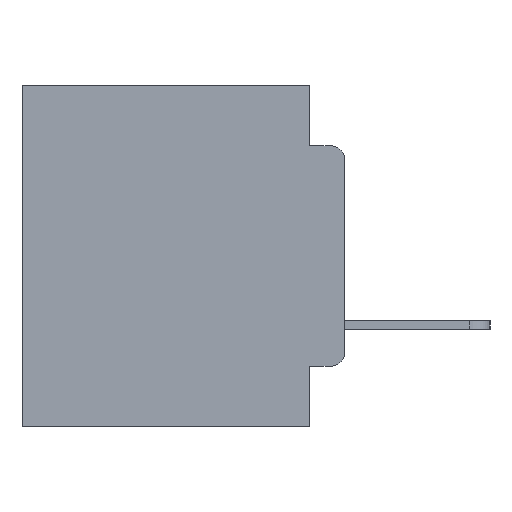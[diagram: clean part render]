
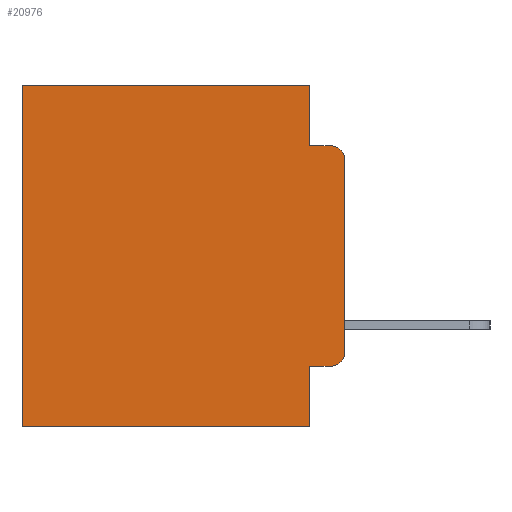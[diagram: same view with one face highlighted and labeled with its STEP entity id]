
A CAD part, left-side view. The second image highlights one B-rep face of the part: STEP entity #20976.
In plain terms, the highlighted planar face has unit normal (-1, 0, 0).
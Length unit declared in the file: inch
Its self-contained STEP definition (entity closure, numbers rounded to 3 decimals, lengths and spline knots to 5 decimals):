
#806 = CARTESIAN_POINT ( 'NONE',  ( 0.298, 0.051, -0.4115 ) ) ;
#814 = EDGE_LOOP ( 'NONE', ( #24958, #14508, #8921, #24069, #3174, #27564, #15172, #28397, #24677, #23780 ) ) ;
#1086 = VERTEX_POINT ( 'NONE', #5333 ) ;
#1125 = LINE ( 'NONE', #21818, #23109 ) ;
#1185 = DIRECTION ( 'NONE',  ( 0., 0., -1. ) ) ;
#1727 = DIRECTION ( 'NONE',  ( 1., 0., 0. ) ) ;
#2518 = CARTESIAN_POINT ( 'NONE',  ( 0.298, 0.051, -0.0885 ) ) ;
#2690 = VECTOR ( 'NONE', #19543, 39.37008 ) ;
#2940 = CARTESIAN_POINT ( 'NONE',  ( 0.298, 0., -0.1085 ) ) ;
#3174 = ORIENTED_EDGE ( 'NONE', *, *, #16804, .T. ) ;
#3252 = CARTESIAN_POINT ( 'NONE',  ( 0.298, 0.051, -0.0885 ) ) ;
#3328 = DIRECTION ( 'NONE',  ( 0., 0., -1. ) ) ;
#3521 = CARTESIAN_POINT ( 'NONE',  ( 0.298, 0., 0. ) ) ;
#3951 = CARTESIAN_POINT ( 'NONE',  ( 0.298, 0., 0. ) ) ;
#4166 = DIRECTION ( 'NONE',  ( 0., 0., -1. ) ) ;
#4371 = DIRECTION ( 'NONE',  ( 0., 1., 0. ) ) ;
#4729 = DIRECTION ( 'NONE',  ( 0., -1., 0. ) ) ;
#4752 = LINE ( 'NONE', #21910, #2690 ) ;
#4951 = EDGE_CURVE ( 'NONE', #8878, #1086, #20096, .T. ) ;
#5032 = DIRECTION ( 'NONE',  ( 0., -1., 0. ) ) ;
#5333 = CARTESIAN_POINT ( 'NONE',  ( 0.298, 0.02, -0.0885 ) ) ;
#6198 = LINE ( 'NONE', #19622, #10331 ) ;
#6362 = EDGE_CURVE ( 'NONE', #19296, #1086, #15864, .T. ) ;
#6628 = VECTOR ( 'NONE', #4371, 39.37008 ) ;
#6692 = EDGE_CURVE ( 'NONE', #16845, #23964, #1125, .T. ) ;
#7140 = AXIS2_PLACEMENT_3D ( 'NONE', #14344, #10156, #1185 ) ;
#7438 = AXIS2_PLACEMENT_3D ( 'NONE', #3951, #1727, #10714 ) ;
#7787 = CARTESIAN_POINT ( 'NONE',  ( 0.298, 0.051, -0.4115 ) ) ;
#7881 = EDGE_CURVE ( 'NONE', #19242, #22658, #18175, .T. ) ;
#8309 = VERTEX_POINT ( 'NONE', #23051 ) ;
#8380 = LINE ( 'NONE', #27489, #21716 ) ;
#8697 = AXIS2_PLACEMENT_3D ( 'NONE', #27974, #12816, #14950 ) ;
#8708 = DIRECTION ( 'NONE',  ( 0., 0., -1. ) ) ;
#8878 = VERTEX_POINT ( 'NONE', #2940 ) ;
#8921 = ORIENTED_EDGE ( 'NONE', *, *, #6362, .F. ) ;
#9061 = VECTOR ( 'NONE', #5032, 39.37008 ) ;
#9118 = FACE_OUTER_BOUND ( 'NONE', #814, .T. ) ;
#9378 = VECTOR ( 'NONE', #4729, 39.37008 ) ;
#10156 = DIRECTION ( 'NONE',  ( -1., 0., 0. ) ) ;
#10197 = EDGE_CURVE ( 'NONE', #8878, #22658, #28335, .T. ) ;
#10331 = VECTOR ( 'NONE', #8708, 39.37008 ) ;
#10714 = DIRECTION ( 'NONE',  ( 0., 0., -1. ) ) ;
#11926 = EDGE_CURVE ( 'NONE', #16845, #19242, #14888, .T. ) ;
#12172 = EDGE_CURVE ( 'NONE', #23964, #8309, #8380, .T. ) ;
#12650 = DIRECTION ( 'NONE',  ( 0., 1., 0. ) ) ;
#12816 = DIRECTION ( 'NONE',  ( -1., 0., 0. ) ) ;
#14344 = CARTESIAN_POINT ( 'NONE',  ( 0.298, 0.02, -0.1085 ) ) ;
#14508 = ORIENTED_EDGE ( 'NONE', *, *, #4951, .T. ) ;
#14625 = VECTOR ( 'NONE', #3328, 39.37008 ) ;
#14888 = LINE ( 'NONE', #806, #9061 ) ;
#14950 = DIRECTION ( 'NONE',  ( 0., 0., -1. ) ) ;
#15172 = ORIENTED_EDGE ( 'NONE', *, *, #12172, .F. ) ;
#15430 = CARTESIAN_POINT ( 'NONE',  ( 0.298, 0., -0.3915 ) ) ;
#15864 = LINE ( 'NONE', #2518, #9378 ) ;
#16404 = VERTEX_POINT ( 'NONE', #23049 ) ;
#16804 = EDGE_CURVE ( 'NONE', #16404, #25342, #20676, .T. ) ;
#16845 = VERTEX_POINT ( 'NONE', #7787 ) ;
#18175 = CIRCLE ( 'NONE', #8697, 0.02 ) ;
#19242 = VERTEX_POINT ( 'NONE', #20844 ) ;
#19296 = VERTEX_POINT ( 'NONE', #3252 ) ;
#19543 = DIRECTION ( 'NONE',  ( 0., 0., -1. ) ) ;
#19622 = CARTESIAN_POINT ( 'NONE',  ( 0.298, 0.473, 0. ) ) ;
#19835 = CARTESIAN_POINT ( 'NONE',  ( 0.298, 0., 0. ) ) ;
#20096 = CIRCLE ( 'NONE', #7140, 0.02 ) ;
#20669 = CARTESIAN_POINT ( 'NONE',  ( 0.298, 0.473, 0. ) ) ;
#20676 = LINE ( 'NONE', #19835, #6628 ) ;
#20844 = CARTESIAN_POINT ( 'NONE',  ( 0.298, 0.02, -0.4115 ) ) ;
#20976 = ADVANCED_FACE ( 'NONE', ( #9118 ), #26073, .F. ) ;
#21716 = VECTOR ( 'NONE', #12650, 39.37008 ) ;
#21818 = CARTESIAN_POINT ( 'NONE',  ( 0.298, 0.051, 0. ) ) ;
#21910 = CARTESIAN_POINT ( 'NONE',  ( 0.298, 0.051, 0. ) ) ;
#22083 = CARTESIAN_POINT ( 'NONE',  ( 0.298, 0.051, -0.5 ) ) ;
#22658 = VERTEX_POINT ( 'NONE', #15430 ) ;
#23049 = CARTESIAN_POINT ( 'NONE',  ( 0.298, 0.051, 0. ) ) ;
#23051 = CARTESIAN_POINT ( 'NONE',  ( 0.298, 0.473, -0.5 ) ) ;
#23109 = VECTOR ( 'NONE', #4166, 39.37008 ) ;
#23780 = ORIENTED_EDGE ( 'NONE', *, *, #7881, .T. ) ;
#23814 = EDGE_CURVE ( 'NONE', #25342, #8309, #6198, .T. ) ;
#23964 = VERTEX_POINT ( 'NONE', #22083 ) ;
#24069 = ORIENTED_EDGE ( 'NONE', *, *, #25019, .F. ) ;
#24677 = ORIENTED_EDGE ( 'NONE', *, *, #11926, .T. ) ;
#24958 = ORIENTED_EDGE ( 'NONE', *, *, #10197, .F. ) ;
#25019 = EDGE_CURVE ( 'NONE', #16404, #19296, #4752, .T. ) ;
#25342 = VERTEX_POINT ( 'NONE', #20669 ) ;
#26073 = PLANE ( 'NONE',  #7438 ) ;
#27489 = CARTESIAN_POINT ( 'NONE',  ( 0.298, 0., -0.5 ) ) ;
#27564 = ORIENTED_EDGE ( 'NONE', *, *, #23814, .T. ) ;
#27974 = CARTESIAN_POINT ( 'NONE',  ( 0.298, 0.02, -0.3915 ) ) ;
#28335 = LINE ( 'NONE', #3521, #14625 ) ;
#28397 = ORIENTED_EDGE ( 'NONE', *, *, #6692, .F. ) ;
